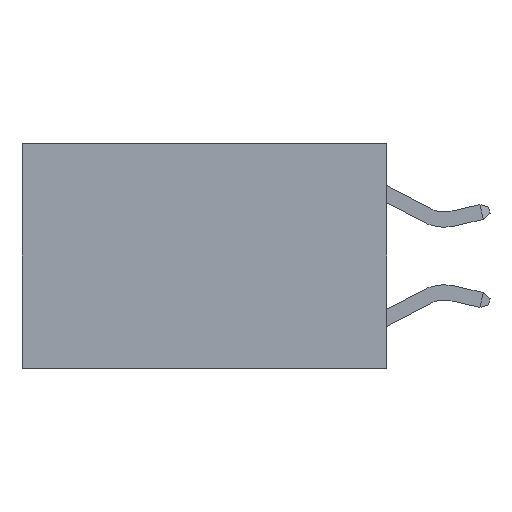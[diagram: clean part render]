
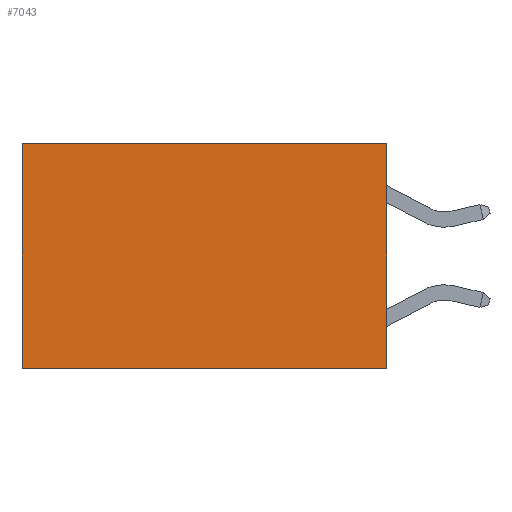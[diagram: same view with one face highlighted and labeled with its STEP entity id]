
A CAD part, left-side view. The second image highlights one B-rep face of the part: STEP entity #7043.
In plain terms, the highlighted planar face has unit normal (-1, 0, 0).
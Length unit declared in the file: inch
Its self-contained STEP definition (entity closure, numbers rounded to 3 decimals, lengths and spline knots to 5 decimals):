
#24 = DIRECTION ( 'NONE',  ( 0., 0., -1. ) ) ;
#125 = CARTESIAN_POINT ( 'NONE',  ( 0.2625, 0., 0. ) ) ;
#446 = PLANE ( 'NONE',  #16187 ) ;
#1605 = LINE ( 'NONE', #15675, #5593 ) ;
#2052 = DIRECTION ( 'NONE',  ( 0., 0., -1. ) ) ;
#4856 = VECTOR ( 'NONE', #14175, 39.37008 ) ;
#5593 = VECTOR ( 'NONE', #15455, 39.37008 ) ;
#6101 = VERTEX_POINT ( 'NONE', #18926 ) ;
#6337 = DIRECTION ( 'NONE',  ( 0., 1., 0. ) ) ;
#6890 = LINE ( 'NONE', #125, #17346 ) ;
#7043 = ADVANCED_FACE ( 'NONE', ( #12399 ), #446, .F. ) ;
#7775 = CARTESIAN_POINT ( 'NONE',  ( 0.2625, 0.6, -0.37 ) ) ;
#8033 = LINE ( 'NONE', #14910, #10957 ) ;
#8227 = ORIENTED_EDGE ( 'NONE', *, *, #14490, .F. ) ;
#8780 = VERTEX_POINT ( 'NONE', #15323 ) ;
#10517 = VERTEX_POINT ( 'NONE', #7775 ) ;
#10599 = CARTESIAN_POINT ( 'NONE',  ( 0.2625, 0., 0. ) ) ;
#10898 = LINE ( 'NONE', #19116, #4856 ) ;
#10957 = VECTOR ( 'NONE', #6337, 39.37008 ) ;
#10965 = ORIENTED_EDGE ( 'NONE', *, *, #15517, .T. ) ;
#12399 = FACE_OUTER_BOUND ( 'NONE', #13350, .T. ) ;
#12564 = EDGE_CURVE ( 'NONE', #6101, #13660, #8033, .T. ) ;
#13350 = EDGE_LOOP ( 'NONE', ( #10965, #20083, #8227, #21857 ) ) ;
#13660 = VERTEX_POINT ( 'NONE', #15088 ) ;
#14175 = DIRECTION ( 'NONE',  ( 0., 1., 0. ) ) ;
#14490 = EDGE_CURVE ( 'NONE', #6101, #8780, #6890, .T. ) ;
#14910 = CARTESIAN_POINT ( 'NONE',  ( 0.2625, 0., 0. ) ) ;
#15053 = EDGE_CURVE ( 'NONE', #8780, #10517, #10898, .T. ) ;
#15088 = CARTESIAN_POINT ( 'NONE',  ( 0.2625, 0.6, 0. ) ) ;
#15323 = CARTESIAN_POINT ( 'NONE',  ( 0.2625, 0., -0.37 ) ) ;
#15455 = DIRECTION ( 'NONE',  ( 0., 0., -1. ) ) ;
#15517 = EDGE_CURVE ( 'NONE', #13660, #10517, #1605, .T. ) ;
#15675 = CARTESIAN_POINT ( 'NONE',  ( 0.2625, 0.6, 0. ) ) ;
#16187 = AXIS2_PLACEMENT_3D ( 'NONE', #10599, #17452, #2052 ) ;
#17346 = VECTOR ( 'NONE', #24, 39.37008 ) ;
#17452 = DIRECTION ( 'NONE',  ( 1., 0., 0. ) ) ;
#18926 = CARTESIAN_POINT ( 'NONE',  ( 0.2625, 0., 0. ) ) ;
#19116 = CARTESIAN_POINT ( 'NONE',  ( 0.2625, 0., -0.37 ) ) ;
#20083 = ORIENTED_EDGE ( 'NONE', *, *, #15053, .F. ) ;
#21857 = ORIENTED_EDGE ( 'NONE', *, *, #12564, .T. ) ;
